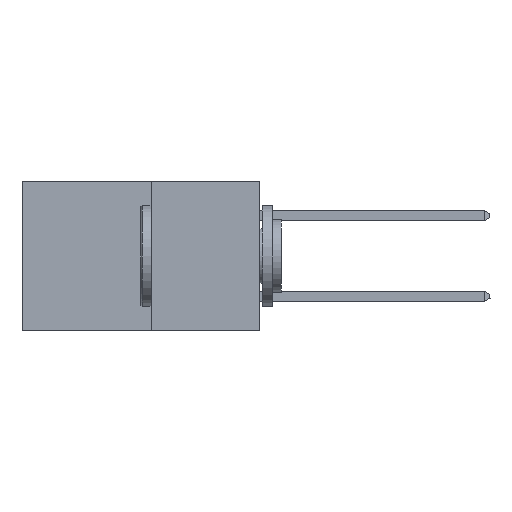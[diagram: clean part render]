
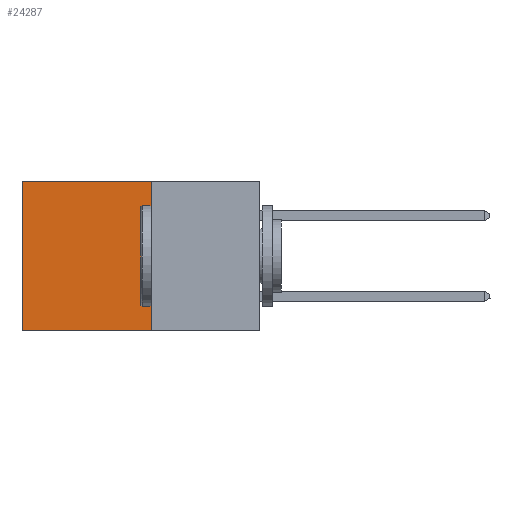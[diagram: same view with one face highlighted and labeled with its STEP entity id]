
A CAD part, left-side view. The second image highlights one B-rep face of the part: STEP entity #24287.
In plain terms, the highlighted planar face has unit normal (-1, 0, 0).
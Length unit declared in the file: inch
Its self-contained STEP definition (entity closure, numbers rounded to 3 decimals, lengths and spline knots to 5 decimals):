
#159 = CARTESIAN_POINT ( 'NONE',  ( 0.277, 0.59, -0.37 ) ) ;
#451 = CARTESIAN_POINT ( 'NONE',  ( 0.277, 0.27, 0. ) ) ;
#656 = EDGE_LOOP ( 'NONE', ( #792, #10097, #14665, #15709 ) ) ;
#792 = ORIENTED_EDGE ( 'NONE', *, *, #27045, .T. ) ;
#1149 = DIRECTION ( 'NONE',  ( 0., 0., -1. ) ) ;
#1451 = VECTOR ( 'NONE', #4504, 39.37008 ) ;
#1821 = CARTESIAN_POINT ( 'NONE',  ( 0.277, 0.59, -0.37 ) ) ;
#2297 = DIRECTION ( 'NONE',  ( 0., 1., 0. ) ) ;
#2754 = LINE ( 'NONE', #159, #20696 ) ;
#3011 = VERTEX_POINT ( 'NONE', #451 ) ;
#3671 = CARTESIAN_POINT ( 'NONE',  ( 0.277, 0.27, 0. ) ) ;
#3818 = EDGE_CURVE ( 'NONE', #3011, #6590, #19426, .T. ) ;
#4039 = VECTOR ( 'NONE', #2297, 39.37008 ) ;
#4332 = LINE ( 'NONE', #6794, #21485 ) ;
#4504 = DIRECTION ( 'NONE',  ( 0., 1., 0. ) ) ;
#6401 = AXIS2_PLACEMENT_3D ( 'NONE', #22111, #15255, #1149 ) ;
#6590 = VERTEX_POINT ( 'NONE', #17065 ) ;
#6794 = CARTESIAN_POINT ( 'NONE',  ( 0.277, 0.27, -0.37 ) ) ;
#10097 = ORIENTED_EDGE ( 'NONE', *, *, #23901, .F. ) ;
#13971 = FACE_OUTER_BOUND ( 'NONE', #656, .T. ) ;
#14385 = DIRECTION ( 'NONE',  ( 0., 0., -1. ) ) ;
#14665 = ORIENTED_EDGE ( 'NONE', *, *, #26122, .F. ) ;
#15255 = DIRECTION ( 'NONE',  ( 1., 0., 0. ) ) ;
#15709 = ORIENTED_EDGE ( 'NONE', *, *, #3818, .T. ) ;
#17065 = CARTESIAN_POINT ( 'NONE',  ( 0.277, 0.59, 0. ) ) ;
#17078 = VERTEX_POINT ( 'NONE', #25582 ) ;
#19426 = LINE ( 'NONE', #3671, #1451 ) ;
#20693 = DIRECTION ( 'NONE',  ( 0., 0., -1. ) ) ;
#20696 = VECTOR ( 'NONE', #14385, 39.37008 ) ;
#21485 = VECTOR ( 'NONE', #20693, 39.37008 ) ;
#22111 = CARTESIAN_POINT ( 'NONE',  ( 0.277, 0.27, -0.37 ) ) ;
#22651 = LINE ( 'NONE', #26578, #4039 ) ;
#23091 = VERTEX_POINT ( 'NONE', #1821 ) ;
#23901 = EDGE_CURVE ( 'NONE', #17078, #23091, #22651, .T. ) ;
#24287 = ADVANCED_FACE ( 'NONE', ( #13971 ), #29083, .F. ) ;
#25582 = CARTESIAN_POINT ( 'NONE',  ( 0.277, 0.27, -0.37 ) ) ;
#26122 = EDGE_CURVE ( 'NONE', #3011, #17078, #4332, .T. ) ;
#26578 = CARTESIAN_POINT ( 'NONE',  ( 0.277, 0.27, -0.37 ) ) ;
#27045 = EDGE_CURVE ( 'NONE', #6590, #23091, #2754, .T. ) ;
#29083 = PLANE ( 'NONE',  #6401 ) ;
